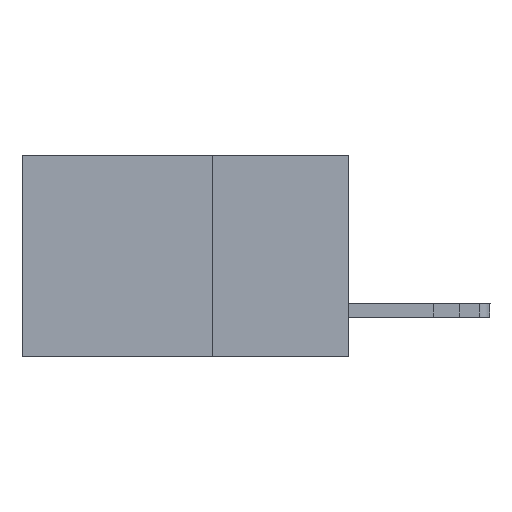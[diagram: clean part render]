
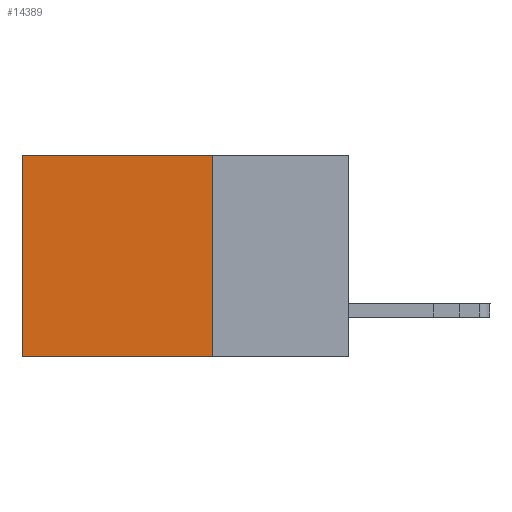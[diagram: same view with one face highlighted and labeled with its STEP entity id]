
A CAD part, left-side view. The second image highlights one B-rep face of the part: STEP entity #14389.
In plain terms, the highlighted planar face has unit normal (-1, 0, 0).
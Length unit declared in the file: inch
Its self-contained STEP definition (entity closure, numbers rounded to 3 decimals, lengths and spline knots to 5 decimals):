
#51 = DIRECTION ( 'NONE',  ( 1., 0., 0. ) ) ;
#228 = VERTEX_POINT ( 'NONE', #15049 ) ;
#1066 = ORIENTED_EDGE ( 'NONE', *, *, #6938, .T. ) ;
#1265 = PLANE ( 'NONE',  #6503 ) ;
#1318 = ORIENTED_EDGE ( 'NONE', *, *, #6809, .F. ) ;
#1353 = VECTOR ( 'NONE', #2845, 39.37008 ) ;
#1500 = EDGE_CURVE ( 'NONE', #11356, #4329, #11545, .T. ) ;
#1755 = DIRECTION ( 'NONE',  ( 0., 0., -1. ) ) ;
#2335 = VERTEX_POINT ( 'NONE', #5463 ) ;
#2452 = CARTESIAN_POINT ( 'NONE',  ( 0.298, 0.25, 0. ) ) ;
#2708 = FACE_OUTER_BOUND ( 'NONE', #8465, .T. ) ;
#2845 = DIRECTION ( 'NONE',  ( 0., 1., 0. ) ) ;
#3295 = CARTESIAN_POINT ( 'NONE',  ( 0.298, 0.6, 0. ) ) ;
#4329 = VERTEX_POINT ( 'NONE', #7747 ) ;
#5463 = CARTESIAN_POINT ( 'NONE',  ( 0.298, 0.6, -0.37 ) ) ;
#6132 = CARTESIAN_POINT ( 'NONE',  ( 0.298, 0.25, 0. ) ) ;
#6503 = AXIS2_PLACEMENT_3D ( 'NONE', #6132, #51, #10998 ) ;
#6699 = VECTOR ( 'NONE', #12025, 39.37008 ) ;
#6809 = EDGE_CURVE ( 'NONE', #4329, #2335, #8443, .T. ) ;
#6837 = ORIENTED_EDGE ( 'NONE', *, *, #14906, .T. ) ;
#6938 = EDGE_CURVE ( 'NONE', #11356, #228, #8605, .T. ) ;
#7602 = ORIENTED_EDGE ( 'NONE', *, *, #1500, .F. ) ;
#7747 = CARTESIAN_POINT ( 'NONE',  ( 0.298, 0.25, -0.37 ) ) ;
#8443 = LINE ( 'NONE', #13287, #6699 ) ;
#8465 = EDGE_LOOP ( 'NONE', ( #6837, #1318, #7602, #1066 ) ) ;
#8605 = LINE ( 'NONE', #9881, #1353 ) ;
#9041 = LINE ( 'NONE', #3295, #13898 ) ;
#9881 = CARTESIAN_POINT ( 'NONE',  ( 0.298, 0.25, 0. ) ) ;
#10560 = DIRECTION ( 'NONE',  ( 0., 0., -1. ) ) ;
#10998 = DIRECTION ( 'NONE',  ( 0., 0., -1. ) ) ;
#11356 = VERTEX_POINT ( 'NONE', #2452 ) ;
#11545 = LINE ( 'NONE', #15293, #14834 ) ;
#12025 = DIRECTION ( 'NONE',  ( 0., 1., 0. ) ) ;
#13287 = CARTESIAN_POINT ( 'NONE',  ( 0.298, 0.25, -0.37 ) ) ;
#13898 = VECTOR ( 'NONE', #10560, 39.37008 ) ;
#14389 = ADVANCED_FACE ( 'NONE', ( #2708 ), #1265, .F. ) ;
#14834 = VECTOR ( 'NONE', #1755, 39.37008 ) ;
#14906 = EDGE_CURVE ( 'NONE', #228, #2335, #9041, .T. ) ;
#15049 = CARTESIAN_POINT ( 'NONE',  ( 0.298, 0.6, 0. ) ) ;
#15293 = CARTESIAN_POINT ( 'NONE',  ( 0.298, 0.25, 0. ) ) ;
